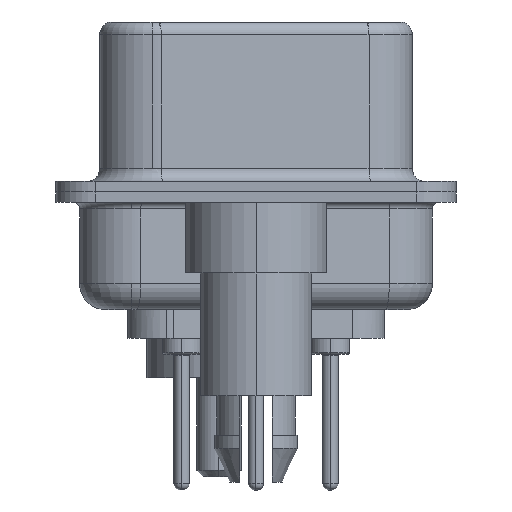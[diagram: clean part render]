
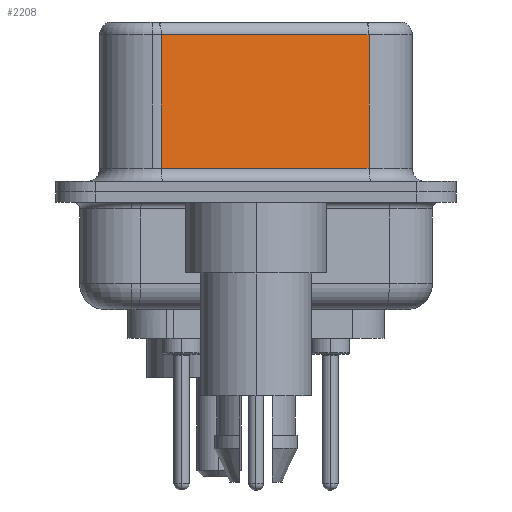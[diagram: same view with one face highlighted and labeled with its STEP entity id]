
A CAD part, left-side view. The second image highlights one B-rep face of the part: STEP entity #2208.
In plain terms, the highlighted planar face has unit normal (-0.985, -0.174, 0).
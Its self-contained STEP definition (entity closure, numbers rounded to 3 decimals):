
#886 = LINE ( 'NONE', #3073, #28268 ) ;
#1705 = CARTESIAN_POINT ( 'NONE',  ( 5.132, -4.322, 6.02 ) ) ;
#2208 = ADVANCED_FACE ( 'NONE', ( #15111 ), #8550, .F. ) ;
#2397 = EDGE_CURVE ( 'NONE', #32440, #30027, #24303, .T. ) ;
#3073 = CARTESIAN_POINT ( 'NONE',  ( 5.132, -4.322, 0.9 ) ) ;
#4036 = DIRECTION ( 'NONE',  ( 0., 0., -1. ) ) ;
#4578 = VECTOR ( 'NONE', #4036, 1000. ) ;
#4678 = CARTESIAN_POINT ( 'NONE',  ( 5.132, -4.322, 6.52 ) ) ;
#6360 = EDGE_CURVE ( 'NONE', #16089, #32053, #12413, .T. ) ;
#8550 = PLANE ( 'NONE',  #14874 ) ;
#10290 = CARTESIAN_POINT ( 'NONE',  ( 3.73, 3.628, 0.9 ) ) ;
#12203 = CARTESIAN_POINT ( 'NONE',  ( 3.73, 3.628, 6.02 ) ) ;
#12413 = LINE ( 'NONE', #4678, #4578 ) ;
#13040 = ORIENTED_EDGE ( 'NONE', *, *, #6360, .F. ) ;
#13702 = DIRECTION ( 'NONE',  ( 0.174, -0.985, 0. ) ) ;
#14849 = EDGE_CURVE ( 'NONE', #16089, #32440, #15542, .T. ) ;
#14874 = AXIS2_PLACEMENT_3D ( 'NONE', #23300, #30860, #15842 ) ;
#15111 = FACE_OUTER_BOUND ( 'NONE', #18624, .T. ) ;
#15364 = CARTESIAN_POINT ( 'NONE',  ( 3.73, 3.628, 6.52 ) ) ;
#15542 = LINE ( 'NONE', #31482, #29714 ) ;
#15842 = DIRECTION ( 'NONE',  ( -0.174, 0.985, 0. ) ) ;
#16089 = VERTEX_POINT ( 'NONE', #1705 ) ;
#17752 = CARTESIAN_POINT ( 'NONE',  ( 5.132, -4.322, 0.9 ) ) ;
#17922 = ORIENTED_EDGE ( 'NONE', *, *, #33127, .T. ) ;
#18624 = EDGE_LOOP ( 'NONE', ( #13040, #31344, #31723, #17922 ) ) ;
#23300 = CARTESIAN_POINT ( 'NONE',  ( 5.132, -4.322, 6.52 ) ) ;
#24303 = LINE ( 'NONE', #15364, #30533 ) ;
#28268 = VECTOR ( 'NONE', #13702, 1000. ) ;
#29714 = VECTOR ( 'NONE', #31359, 1000. ) ;
#30027 = VERTEX_POINT ( 'NONE', #10290 ) ;
#30533 = VECTOR ( 'NONE', #30654, 1000. ) ;
#30654 = DIRECTION ( 'NONE',  ( 0., 0., -1. ) ) ;
#30860 = DIRECTION ( 'NONE',  ( 0.985, 0.174, 0. ) ) ;
#31344 = ORIENTED_EDGE ( 'NONE', *, *, #14849, .T. ) ;
#31359 = DIRECTION ( 'NONE',  ( -0.174, 0.985, 0. ) ) ;
#31482 = CARTESIAN_POINT ( 'NONE',  ( 5.132, -4.322, 6.02 ) ) ;
#31723 = ORIENTED_EDGE ( 'NONE', *, *, #2397, .T. ) ;
#32053 = VERTEX_POINT ( 'NONE', #17752 ) ;
#32440 = VERTEX_POINT ( 'NONE', #12203 ) ;
#33127 = EDGE_CURVE ( 'NONE', #30027, #32053, #886, .T. ) ;
